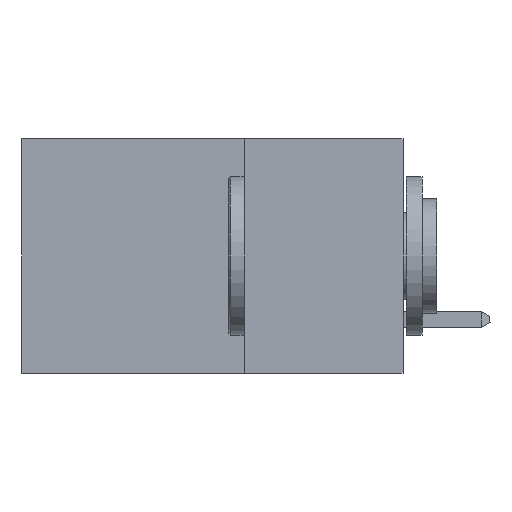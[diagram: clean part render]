
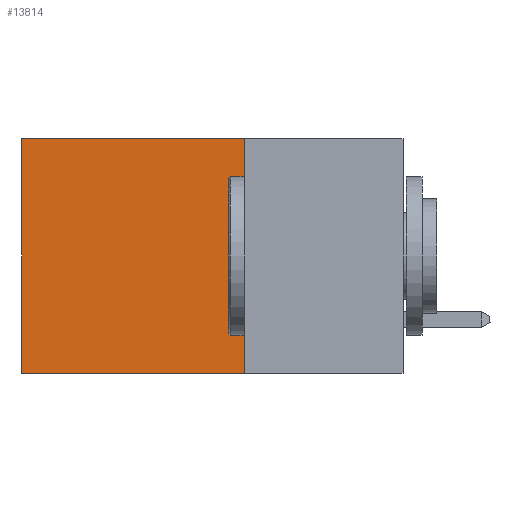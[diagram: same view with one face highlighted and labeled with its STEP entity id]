
A CAD part, left-side view. The second image highlights one B-rep face of the part: STEP entity #13814.
In plain terms, the highlighted planar face has unit normal (-1, 0, 0).
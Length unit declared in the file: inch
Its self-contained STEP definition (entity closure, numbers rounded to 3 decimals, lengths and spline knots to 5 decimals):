
#609 = CARTESIAN_POINT ( 'NONE',  ( 0.2875, 0.25, 0. ) ) ;
#1585 = ORIENTED_EDGE ( 'NONE', *, *, #43183, .F. ) ;
#1675 = ORIENTED_EDGE ( 'NONE', *, *, #42288, .T. ) ;
#1676 = VECTOR ( 'NONE', #20550, 39.37008 ) ;
#3126 = VERTEX_POINT ( 'NONE', #3650 ) ;
#3650 = CARTESIAN_POINT ( 'NONE',  ( 0.2875, 0.25, -0.37 ) ) ;
#4048 = DIRECTION ( 'NONE',  ( 0., 0., -1. ) ) ;
#4192 = DIRECTION ( 'NONE',  ( 1., 0., 0. ) ) ;
#8193 = VECTOR ( 'NONE', #42114, 39.37008 ) ;
#11019 = LINE ( 'NONE', #31387, #1676 ) ;
#12003 = LINE ( 'NONE', #21444, #25675 ) ;
#12316 = DIRECTION ( 'NONE',  ( 0., 1., 0. ) ) ;
#13814 = ADVANCED_FACE ( 'NONE', ( #42397 ), #24973, .F. ) ;
#14761 = LINE ( 'NONE', #37500, #22972 ) ;
#16554 = EDGE_LOOP ( 'NONE', ( #1675, #24432, #1585, #20668 ) ) ;
#16962 = AXIS2_PLACEMENT_3D ( 'NONE', #609, #4192, #4048 ) ;
#17769 = CARTESIAN_POINT ( 'NONE',  ( 0.2875, 0.6, -0.37 ) ) ;
#18233 = CARTESIAN_POINT ( 'NONE',  ( 0.2875, 0.6, 0. ) ) ;
#20550 = DIRECTION ( 'NONE',  ( 0., 1., 0. ) ) ;
#20668 = ORIENTED_EDGE ( 'NONE', *, *, #31683, .T. ) ;
#20892 = CARTESIAN_POINT ( 'NONE',  ( 0.2875, 0.6, 0. ) ) ;
#21444 = CARTESIAN_POINT ( 'NONE',  ( 0.2875, 0.25, -0.37 ) ) ;
#22972 = VECTOR ( 'NONE', #44370, 39.37008 ) ;
#24432 = ORIENTED_EDGE ( 'NONE', *, *, #42429, .F. ) ;
#24973 = PLANE ( 'NONE',  #16962 ) ;
#25287 = VERTEX_POINT ( 'NONE', #43280 ) ;
#25675 = VECTOR ( 'NONE', #12316, 39.37008 ) ;
#26838 = VERTEX_POINT ( 'NONE', #17769 ) ;
#31387 = CARTESIAN_POINT ( 'NONE',  ( 0.2875, 0.25, 0. ) ) ;
#31683 = EDGE_CURVE ( 'NONE', #25287, #42386, #11019, .T. ) ;
#32221 = LINE ( 'NONE', #20892, #8193 ) ;
#37500 = CARTESIAN_POINT ( 'NONE',  ( 0.2875, 0.25, 0. ) ) ;
#42114 = DIRECTION ( 'NONE',  ( 0., 0., -1. ) ) ;
#42288 = EDGE_CURVE ( 'NONE', #42386, #26838, #32221, .T. ) ;
#42386 = VERTEX_POINT ( 'NONE', #18233 ) ;
#42397 = FACE_OUTER_BOUND ( 'NONE', #16554, .T. ) ;
#42429 = EDGE_CURVE ( 'NONE', #3126, #26838, #12003, .T. ) ;
#43183 = EDGE_CURVE ( 'NONE', #25287, #3126, #14761, .T. ) ;
#43280 = CARTESIAN_POINT ( 'NONE',  ( 0.2875, 0.25, 0. ) ) ;
#44370 = DIRECTION ( 'NONE',  ( 0., 0., -1. ) ) ;
